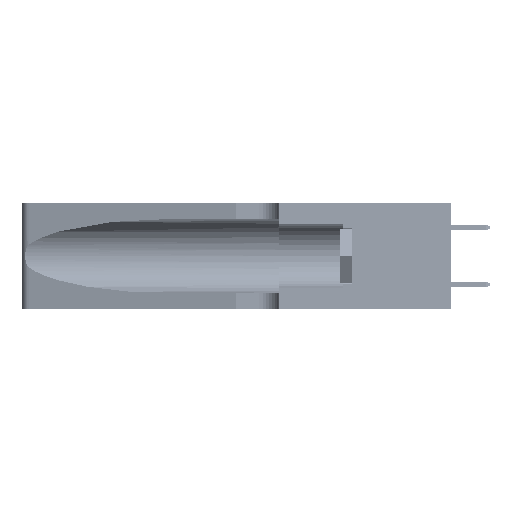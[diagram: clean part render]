
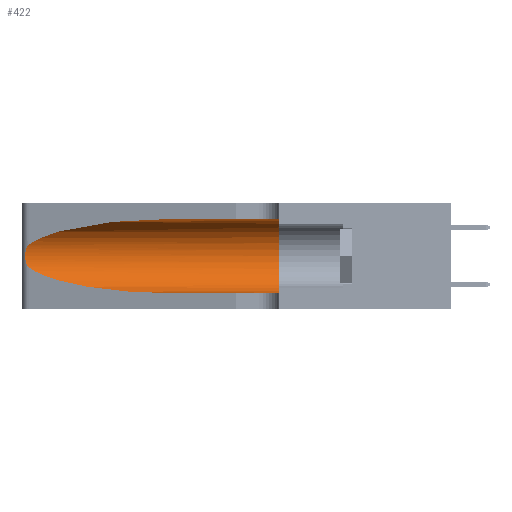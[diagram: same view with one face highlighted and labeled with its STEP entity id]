
A CAD part, left-side view. The second image highlights one B-rep face of the part: STEP entity #422.
In plain terms, the highlighted cylindrical face has radius 3.308 mm (diameter 6.617 mm), a partial arc.
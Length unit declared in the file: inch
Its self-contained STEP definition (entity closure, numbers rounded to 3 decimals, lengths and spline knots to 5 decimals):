
#156 = ORIENTED_EDGE ( 'NONE', *, *, #12653, .T. ) ;
#422 = ADVANCED_FACE ( 'NONE', ( #25719 ), #38266, .F. ) ;
#1385 = AXIS2_PLACEMENT_3D ( 'NONE', #24989, #46002, #28536 ) ;
#1446 = B_SPLINE_CURVE_WITH_KNOTS ( 'NONE', 3,
 ( #50339, #29571, #16978, #16177, #32869, #53918, #20816, #45419, #29315, #16437, #24673, #3586, #7976, #8790 ),
 .UNSPECIFIED., .F., .F.,
 ( 4, 2, 2, 2, 2, 2, 4 ),
 ( 0., 0.00027, 0.00053, 0.00107, 0.0016, 0.00187, 0.00214 ),
 .UNSPECIFIED. ) ;
#2502 = ORIENTED_EDGE ( 'NONE', *, *, #13869, .F. ) ;
#3170 = LINE ( 'NONE', #32189, #31841 ) ;
#3182 = EDGE_CURVE ( 'NONE', #36887, #22983, #32444, .T. ) ;
#3586 = CARTESIAN_POINT ( 'NONE',  ( 0.25639, 1.23186, 0.15144 ) ) ;
#5707 = ORIENTED_EDGE ( 'NONE', *, *, #48783, .F. ) ;
#7504 = CIRCLE ( 'NONE', #1385, 0.13025 ) ;
#7920 = AXIS2_PLACEMENT_3D ( 'NONE', #50568, #42109, #13116 ) ;
#7976 = CARTESIAN_POINT ( 'NONE',  ( 0.25555, 1.22993, 0.14849 ) ) ;
#8790 = CARTESIAN_POINT ( 'NONE',  ( 0.25487, 1.22718, 0.14631 ) ) ;
#10768 = CARTESIAN_POINT ( 'NONE',  ( 0.25487, 1.22718, 0.22369 ) ) ;
#11625 = CARTESIAN_POINT ( 'NONE',  ( 0.25487, 1.22718, 0.14631 ) ) ;
#11669 = DIRECTION ( 'NONE',  ( 0., -1., 0. ) ) ;
#12653 = EDGE_CURVE ( 'NONE', #26473, #33289, #32019, .T. ) ;
#12755 = CARTESIAN_POINT ( 'NONE',  ( 0.1305, 0.72297, 0.05475 ) ) ;
#13116 = DIRECTION ( 'NONE',  ( 0., 0., -1. ) ) ;
#13869 = EDGE_CURVE ( 'NONE', #36887, #50964, #45180, .T. ) ;
#16177 = CARTESIAN_POINT ( 'NONE',  ( 0.25787, 1.23484, 0.2124 ) ) ;
#16437 = CARTESIAN_POINT ( 'NONE',  ( 0.25856, 1.23593, 0.16098 ) ) ;
#16978 = CARTESIAN_POINT ( 'NONE',  ( 0.25639, 1.23184, 0.21858 ) ) ;
#18470 = CARTESIAN_POINT ( 'NONE',  ( 0.1305, 0.72297, 0.31525 ) ) ;
#20602 = CARTESIAN_POINT ( 'NONE',  ( 0.1305, 1.61858, 0.31525 ) ) ;
#20816 = CARTESIAN_POINT ( 'NONE',  ( 0.26075, 1.23896, 0.19203 ) ) ;
#20837 = CARTESIAN_POINT ( 'NONE',  ( 0.1305, 0.72297, 0.05475 ) ) ;
#22983 = VERTEX_POINT ( 'NONE', #10768 ) ;
#24097 = ORIENTED_EDGE ( 'NONE', *, *, #40609, .T. ) ;
#24673 = CARTESIAN_POINT ( 'NONE',  ( 0.25789, 1.23486, 0.15765 ) ) ;
#24989 = CARTESIAN_POINT ( 'NONE',  ( 0.1305, 0.35, 0.185 ) ) ;
#25719 = FACE_OUTER_BOUND ( 'NONE', #39454, .T. ) ;
#26473 = VERTEX_POINT ( 'NONE', #11625 ) ;
#26693 = CARTESIAN_POINT ( 'NONE',  ( 0.25487, 1.22718, 0.22369 ) ) ;
#26816 = VERTEX_POINT ( 'NONE', #30466 ) ;
#28536 = DIRECTION ( 'NONE',  ( 0., 0., 1. ) ) ;
#29315 = CARTESIAN_POINT ( 'NONE',  ( 0.26017, 1.23833, 0.17102 ) ) ;
#29571 = CARTESIAN_POINT ( 'NONE',  ( 0.25555, 1.22994, 0.2215 ) ) ;
#29834 = ORIENTED_EDGE ( 'NONE', *, *, #45027, .T. ) ;
#30466 = CARTESIAN_POINT ( 'NONE',  ( 0.1305, 0.35, 0.05475 ) ) ;
#30523 = CARTESIAN_POINT ( 'NONE',  ( 0.2373, 1.15595, 0.28018 ) ) ;
#31841 = VECTOR ( 'NONE', #11669, 39.37008 ) ;
#32019 =( BOUNDED_CURVE ( )  B_SPLINE_CURVE ( 3, ( #33435, #47034, #33691, #20837 ),
 .UNSPECIFIED., .F., .T. ) 
 B_SPLINE_CURVE_WITH_KNOTS ( ( 4, 4 ),
 ( 3.44316, 4.71239 ),
 .UNSPECIFIED. ) 
 CURVE ( )  GEOMETRIC_REPRESENTATION_ITEM ( )  RATIONAL_B_SPLINE_CURVE ( ( 1., 0.87, 0.87, 1. ) ) 
 REPRESENTATION_ITEM ( '' )  );
#32103 = DIRECTION ( 'NONE',  ( 0., -1., 0. ) ) ;
#32189 = CARTESIAN_POINT ( 'NONE',  ( 0.1305, 1.61858, 0.05475 ) ) ;
#32444 =( BOUNDED_CURVE ( )  B_SPLINE_CURVE ( 3, ( #18470, #47439, #30523, #26693 ),
 .UNSPECIFIED., .F., .T. ) 
 B_SPLINE_CURVE_WITH_KNOTS ( ( 4, 4 ),
 ( 1.5708, 2.84003 ),
 .UNSPECIFIED. ) 
 CURVE ( )  GEOMETRIC_REPRESENTATION_ITEM ( )  RATIONAL_B_SPLINE_CURVE ( ( 1., 0.87, 0.87, 1. ) ) 
 REPRESENTATION_ITEM ( '' )  );
#32869 = CARTESIAN_POINT ( 'NONE',  ( 0.25854, 1.2359, 0.20912 ) ) ;
#33289 = VERTEX_POINT ( 'NONE', #12755 ) ;
#33435 = CARTESIAN_POINT ( 'NONE',  ( 0.25487, 1.22718, 0.14631 ) ) ;
#33691 = CARTESIAN_POINT ( 'NONE',  ( 0.18966, 0.96281, 0.05475 ) ) ;
#36337 = ORIENTED_EDGE ( 'NONE', *, *, #3182, .T. ) ;
#36348 = CARTESIAN_POINT ( 'NONE',  ( 0.1305, 0.35, 0.31525 ) ) ;
#36887 = VERTEX_POINT ( 'NONE', #42786 ) ;
#38266 = CYLINDRICAL_SURFACE ( 'NONE', #7920, 0.13025 ) ;
#39454 = EDGE_LOOP ( 'NONE', ( #36337, #24097, #156, #29834, #5707, #2502 ) ) ;
#40609 = EDGE_CURVE ( 'NONE', #22983, #26473, #1446, .T. ) ;
#42109 = DIRECTION ( 'NONE',  ( 0., -1., 0. ) ) ;
#42786 = CARTESIAN_POINT ( 'NONE',  ( 0.1305, 0.72297, 0.31525 ) ) ;
#45027 = EDGE_CURVE ( 'NONE', #33289, #26816, #3170, .T. ) ;
#45180 = LINE ( 'NONE', #20602, #49901 ) ;
#45419 = CARTESIAN_POINT ( 'NONE',  ( 0.26075, 1.23896, 0.178 ) ) ;
#46002 = DIRECTION ( 'NONE',  ( 0., 1., 0. ) ) ;
#47034 = CARTESIAN_POINT ( 'NONE',  ( 0.2373, 1.15595, 0.08982 ) ) ;
#47439 = CARTESIAN_POINT ( 'NONE',  ( 0.18966, 0.96281, 0.31525 ) ) ;
#48783 = EDGE_CURVE ( 'NONE', #50964, #26816, #7504, .T. ) ;
#49901 = VECTOR ( 'NONE', #32103, 39.37008 ) ;
#50339 = CARTESIAN_POINT ( 'NONE',  ( 0.25487, 1.22718, 0.22369 ) ) ;
#50568 = CARTESIAN_POINT ( 'NONE',  ( 0.1305, 1.61858, 0.185 ) ) ;
#50964 = VERTEX_POINT ( 'NONE', #36348 ) ;
#53918 = CARTESIAN_POINT ( 'NONE',  ( 0.26018, 1.23835, 0.19895 ) ) ;
